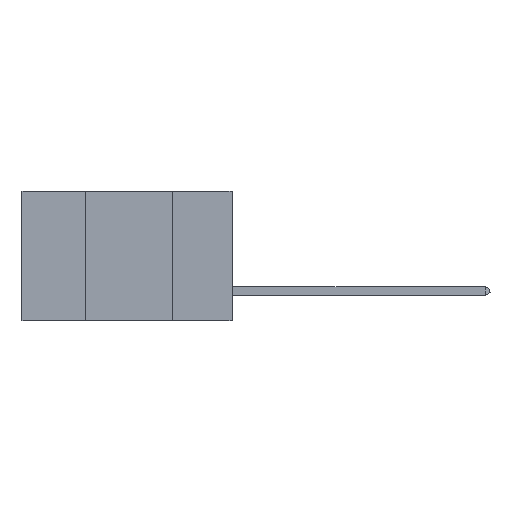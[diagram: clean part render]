
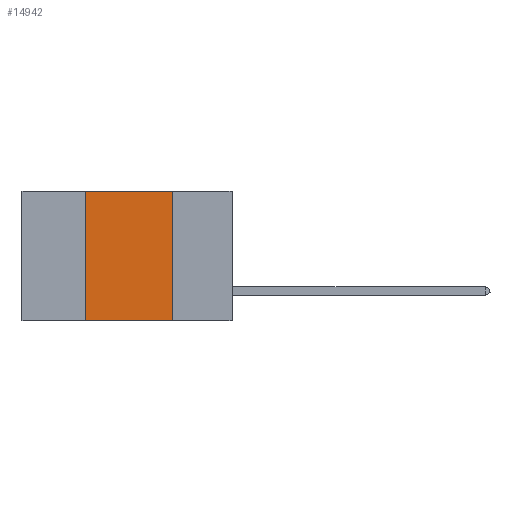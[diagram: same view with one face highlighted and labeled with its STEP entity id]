
A CAD part, left-side view. The second image highlights one B-rep face of the part: STEP entity #14942.
In plain terms, the highlighted planar face has unit normal (-1, 0, 0).
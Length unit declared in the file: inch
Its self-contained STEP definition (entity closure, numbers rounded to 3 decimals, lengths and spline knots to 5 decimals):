
#83 = DIRECTION ( 'NONE',  ( 0., 0., 1. ) ) ;
#1498 = EDGE_LOOP ( 'NONE', ( #3516, #6566, #5675, #14663 ) ) ;
#1986 = CARTESIAN_POINT ( 'NONE',  ( 0., 0.17, -0.37 ) ) ;
#2693 = EDGE_CURVE ( 'NONE', #7787, #7218, #8171, .T. ) ;
#3067 = DIRECTION ( 'NONE',  ( 1., 0., 0. ) ) ;
#3318 = VERTEX_POINT ( 'NONE', #4452 ) ;
#3516 = ORIENTED_EDGE ( 'NONE', *, *, #17157, .F. ) ;
#3626 = EDGE_CURVE ( 'NONE', #7787, #3318, #16834, .T. ) ;
#4093 = VECTOR ( 'NONE', #83, 39.37008 ) ;
#4130 = CARTESIAN_POINT ( 'NONE',  ( 0., 0.17, 0. ) ) ;
#4452 = CARTESIAN_POINT ( 'NONE',  ( 0., 0.42, 0. ) ) ;
#5458 = DIRECTION ( 'NONE',  ( 0., -1., 0. ) ) ;
#5675 = ORIENTED_EDGE ( 'NONE', *, *, #3626, .F. ) ;
#5954 = VECTOR ( 'NONE', #12325, 39.37008 ) ;
#6416 = EDGE_CURVE ( 'NONE', #3318, #15699, #18075, .T. ) ;
#6566 = ORIENTED_EDGE ( 'NONE', *, *, #6416, .F. ) ;
#6916 = VECTOR ( 'NONE', #11155, 39.37008 ) ;
#7218 = VERTEX_POINT ( 'NONE', #1986 ) ;
#7787 = VERTEX_POINT ( 'NONE', #17130 ) ;
#8151 = DIRECTION ( 'NONE',  ( 0., 0., -1. ) ) ;
#8171 = LINE ( 'NONE', #18607, #8665 ) ;
#8665 = VECTOR ( 'NONE', #5458, 39.37008 ) ;
#8945 = AXIS2_PLACEMENT_3D ( 'NONE', #10471, #3067, #8151 ) ;
#9561 = CARTESIAN_POINT ( 'NONE',  ( 0., 0.42, 0. ) ) ;
#10471 = CARTESIAN_POINT ( 'NONE',  ( 0., 0.6, 0. ) ) ;
#11155 = DIRECTION ( 'NONE',  ( 0., 0., -1. ) ) ;
#12325 = DIRECTION ( 'NONE',  ( 0., -1., 0. ) ) ;
#14509 = CARTESIAN_POINT ( 'NONE',  ( 0., 0.17, 0. ) ) ;
#14663 = ORIENTED_EDGE ( 'NONE', *, *, #2693, .T. ) ;
#14942 = ADVANCED_FACE ( 'NONE', ( #16216 ), #17761, .F. ) ;
#15192 = CARTESIAN_POINT ( 'NONE',  ( 0., 0.6, 0. ) ) ;
#15568 = LINE ( 'NONE', #4130, #6916 ) ;
#15699 = VERTEX_POINT ( 'NONE', #14509 ) ;
#16216 = FACE_OUTER_BOUND ( 'NONE', #1498, .T. ) ;
#16834 = LINE ( 'NONE', #9561, #4093 ) ;
#17130 = CARTESIAN_POINT ( 'NONE',  ( 0., 0.42, -0.37 ) ) ;
#17157 = EDGE_CURVE ( 'NONE', #15699, #7218, #15568, .T. ) ;
#17761 = PLANE ( 'NONE',  #8945 ) ;
#18075 = LINE ( 'NONE', #15192, #5954 ) ;
#18607 = CARTESIAN_POINT ( 'NONE',  ( 0., 0.6, -0.37 ) ) ;
